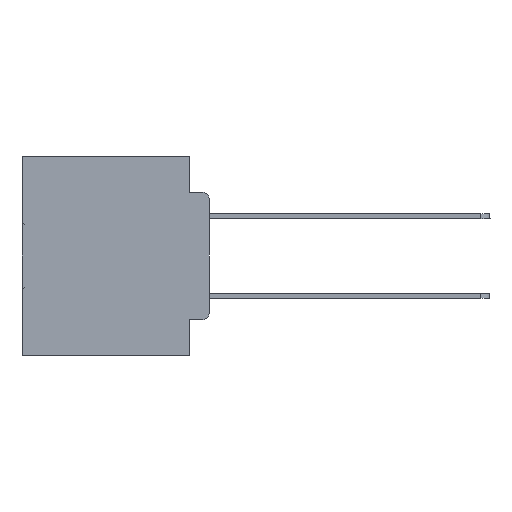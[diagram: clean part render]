
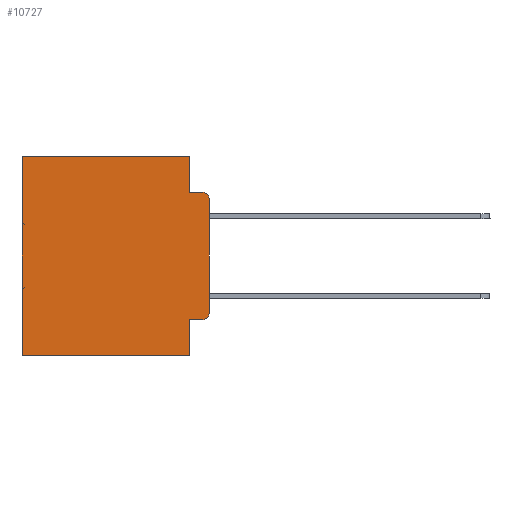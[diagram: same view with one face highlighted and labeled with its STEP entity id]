
A CAD part, left-side view. The second image highlights one B-rep face of the part: STEP entity #10727.
In plain terms, the highlighted planar face has unit normal (-1, 0, 0).
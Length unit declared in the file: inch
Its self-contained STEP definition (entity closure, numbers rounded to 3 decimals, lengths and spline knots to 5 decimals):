
#121 = CARTESIAN_POINT ( 'NONE',  ( 0.298, 0.051, 0. ) ) ;
#126 = EDGE_CURVE ( 'NONE', #1001, #30429, #8228, .T. ) ;
#464 = CARTESIAN_POINT ( 'NONE',  ( 0.298, 0.051, -0.0885 ) ) ;
#1001 = VERTEX_POINT ( 'NONE', #28613 ) ;
#1219 = CARTESIAN_POINT ( 'NONE',  ( 0.298, 0.051, 0. ) ) ;
#1362 = VECTOR ( 'NONE', #5871, 39.37008 ) ;
#1737 = ORIENTED_EDGE ( 'NONE', *, *, #126, .T. ) ;
#2116 = CARTESIAN_POINT ( 'NONE',  ( 0.298, 0., -0.5 ) ) ;
#2513 = ORIENTED_EDGE ( 'NONE', *, *, #26939, .T. ) ;
#2531 = VERTEX_POINT ( 'NONE', #11509 ) ;
#4812 = VERTEX_POINT ( 'NONE', #464 ) ;
#5322 = VECTOR ( 'NONE', #28720, 39.37008 ) ;
#5871 = DIRECTION ( 'NONE',  ( 0., 0., -1. ) ) ;
#6539 = CARTESIAN_POINT ( 'NONE',  ( 0.298, 0.473, 0. ) ) ;
#6642 = CIRCLE ( 'NONE', #17769, 0.02 ) ;
#7293 = LINE ( 'NONE', #13731, #1362 ) ;
#7380 = DIRECTION ( 'NONE',  ( 0., 0., -1. ) ) ;
#7406 = CARTESIAN_POINT ( 'NONE',  ( 0.298, 0.051, -0.5 ) ) ;
#7528 = ORIENTED_EDGE ( 'NONE', *, *, #15050, .F. ) ;
#7808 = DIRECTION ( 'NONE',  ( 0., 1., 0. ) ) ;
#7830 = CARTESIAN_POINT ( 'NONE',  ( 0.298, 0.02, -0.1085 ) ) ;
#7954 = DIRECTION ( 'NONE',  ( 0., 0., -1. ) ) ;
#7967 = ORIENTED_EDGE ( 'NONE', *, *, #15604, .T. ) ;
#8228 = LINE ( 'NONE', #11333, #33543 ) ;
#8271 = EDGE_CURVE ( 'NONE', #13904, #2531, #7293, .T. ) ;
#10305 = LINE ( 'NONE', #11563, #24882 ) ;
#10727 = ADVANCED_FACE ( 'NONE', ( #26681 ), #23835, .F. ) ;
#11139 = EDGE_LOOP ( 'NONE', ( #23423, #2513, #17403, #16596, #1737, #19074, #7528, #25441, #15746, #7967 ) ) ;
#11147 = VECTOR ( 'NONE', #14910, 39.37008 ) ;
#11280 = VERTEX_POINT ( 'NONE', #15175 ) ;
#11333 = CARTESIAN_POINT ( 'NONE',  ( 0.298, 0., 0. ) ) ;
#11509 = CARTESIAN_POINT ( 'NONE',  ( 0.298, 0., -0.3915 ) ) ;
#11563 = CARTESIAN_POINT ( 'NONE',  ( 0.298, 0.051, -0.4115 ) ) ;
#12288 = DIRECTION ( 'NONE',  ( 0., -1., 0. ) ) ;
#13142 = AXIS2_PLACEMENT_3D ( 'NONE', #26314, #23445, #31703 ) ;
#13672 = CARTESIAN_POINT ( 'NONE',  ( 0.298, 0.473, 0. ) ) ;
#13731 = CARTESIAN_POINT ( 'NONE',  ( 0.298, 0., 0. ) ) ;
#13904 = VERTEX_POINT ( 'NONE', #31691 ) ;
#14910 = DIRECTION ( 'NONE',  ( 0., 0., -1. ) ) ;
#14944 = VECTOR ( 'NONE', #12288, 39.37008 ) ;
#15050 = EDGE_CURVE ( 'NONE', #30235, #21972, #22767, .T. ) ;
#15175 = CARTESIAN_POINT ( 'NONE',  ( 0.298, 0.051, -0.4115 ) ) ;
#15604 = EDGE_CURVE ( 'NONE', #30928, #2531, #28675, .T. ) ;
#15746 = ORIENTED_EDGE ( 'NONE', *, *, #35382, .T. ) ;
#16596 = ORIENTED_EDGE ( 'NONE', *, *, #19758, .F. ) ;
#17403 = ORIENTED_EDGE ( 'NONE', *, *, #24676, .F. ) ;
#17769 = AXIS2_PLACEMENT_3D ( 'NONE', #7830, #35179, #7954 ) ;
#18367 = LINE ( 'NONE', #23196, #14944 ) ;
#19074 = ORIENTED_EDGE ( 'NONE', *, *, #26768, .T. ) ;
#19758 = EDGE_CURVE ( 'NONE', #1001, #4812, #20162, .T. ) ;
#20162 = LINE ( 'NONE', #121, #11147 ) ;
#20586 = CARTESIAN_POINT ( 'NONE',  ( 0.298, 0.02, -0.0885 ) ) ;
#21339 = DIRECTION ( 'NONE',  ( 0., 1., 0. ) ) ;
#21408 = CARTESIAN_POINT ( 'NONE',  ( 0.298, 0.473, -0.5 ) ) ;
#21972 = VERTEX_POINT ( 'NONE', #21408 ) ;
#22767 = LINE ( 'NONE', #2116, #33857 ) ;
#22831 = DIRECTION ( 'NONE',  ( 0., -1., 0. ) ) ;
#23196 = CARTESIAN_POINT ( 'NONE',  ( 0.298, 0.051, -0.0885 ) ) ;
#23423 = ORIENTED_EDGE ( 'NONE', *, *, #8271, .F. ) ;
#23445 = DIRECTION ( 'NONE',  ( -1., 0., 0. ) ) ;
#23604 = CARTESIAN_POINT ( 'NONE',  ( 0.298, 0., 0. ) ) ;
#23835 = PLANE ( 'NONE',  #33204 ) ;
#24676 = EDGE_CURVE ( 'NONE', #4812, #32969, #18367, .T. ) ;
#24882 = VECTOR ( 'NONE', #22831, 39.37008 ) ;
#25441 = ORIENTED_EDGE ( 'NONE', *, *, #31372, .F. ) ;
#26276 = DIRECTION ( 'NONE',  ( 0., 0., -1. ) ) ;
#26314 = CARTESIAN_POINT ( 'NONE',  ( 0.298, 0.02, -0.3915 ) ) ;
#26681 = FACE_OUTER_BOUND ( 'NONE', #11139, .T. ) ;
#26768 = EDGE_CURVE ( 'NONE', #30429, #21972, #30699, .T. ) ;
#26912 = CARTESIAN_POINT ( 'NONE',  ( 0.298, 0.02, -0.4115 ) ) ;
#26939 = EDGE_CURVE ( 'NONE', #13904, #32969, #6642, .T. ) ;
#28613 = CARTESIAN_POINT ( 'NONE',  ( 0.298, 0.051, 0. ) ) ;
#28675 = CIRCLE ( 'NONE', #13142, 0.02 ) ;
#28720 = DIRECTION ( 'NONE',  ( 0., 0., -1. ) ) ;
#29398 = VECTOR ( 'NONE', #26276, 39.37008 ) ;
#30235 = VERTEX_POINT ( 'NONE', #7406 ) ;
#30429 = VERTEX_POINT ( 'NONE', #13672 ) ;
#30699 = LINE ( 'NONE', #6539, #5322 ) ;
#30928 = VERTEX_POINT ( 'NONE', #26912 ) ;
#31372 = EDGE_CURVE ( 'NONE', #11280, #30235, #34979, .T. ) ;
#31691 = CARTESIAN_POINT ( 'NONE',  ( 0.298, 0., -0.1085 ) ) ;
#31703 = DIRECTION ( 'NONE',  ( 0., 0., -1. ) ) ;
#31850 = DIRECTION ( 'NONE',  ( 1., 0., 0. ) ) ;
#32969 = VERTEX_POINT ( 'NONE', #20586 ) ;
#33204 = AXIS2_PLACEMENT_3D ( 'NONE', #23604, #31850, #7380 ) ;
#33543 = VECTOR ( 'NONE', #7808, 39.37008 ) ;
#33857 = VECTOR ( 'NONE', #21339, 39.37008 ) ;
#34979 = LINE ( 'NONE', #1219, #29398 ) ;
#35179 = DIRECTION ( 'NONE',  ( -1., 0., 0. ) ) ;
#35382 = EDGE_CURVE ( 'NONE', #11280, #30928, #10305, .T. ) ;
